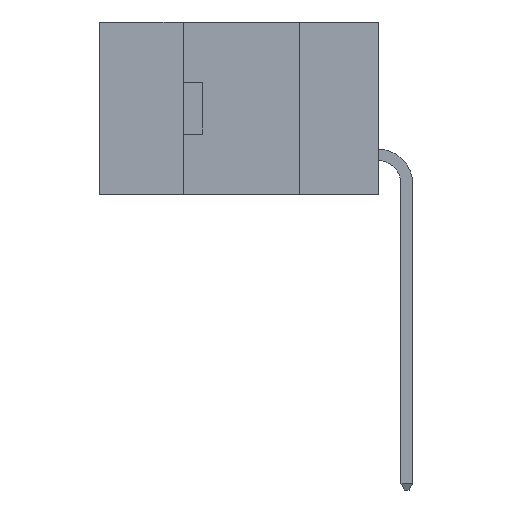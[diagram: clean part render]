
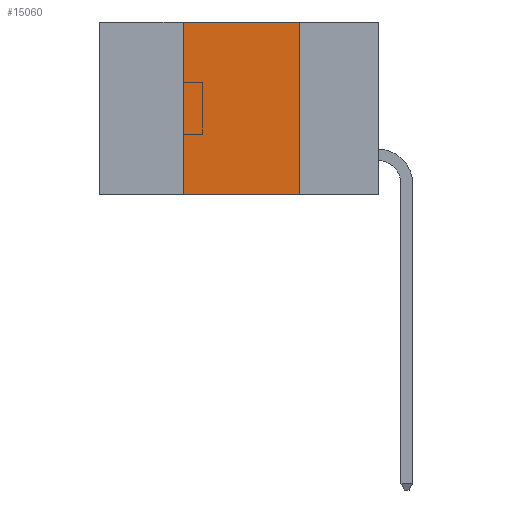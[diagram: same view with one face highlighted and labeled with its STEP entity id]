
A CAD part, left-side view. The second image highlights one B-rep face of the part: STEP entity #15060.
In plain terms, the highlighted planar face has unit normal (-1, 0, 0).
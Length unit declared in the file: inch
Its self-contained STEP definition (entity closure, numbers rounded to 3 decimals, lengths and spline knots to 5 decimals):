
#1055 = CARTESIAN_POINT ( 'NONE',  ( 0., 0.17, 0. ) ) ;
#1073 = DIRECTION ( 'NONE',  ( 0., 0., 1. ) ) ;
#2686 = LINE ( 'NONE', #26273, #6857 ) ;
#3085 = LINE ( 'NONE', #21431, #13430 ) ;
#3296 = FACE_OUTER_BOUND ( 'NONE', #6291, .T. ) ;
#3690 = ORIENTED_EDGE ( 'NONE', *, *, #23099, .T. ) ;
#4072 = VECTOR ( 'NONE', #1073, 39.37008 ) ;
#4460 = EDGE_CURVE ( 'NONE', #14767, #19851, #20591, .T. ) ;
#4537 = DIRECTION ( 'NONE',  ( 0., 0., -1. ) ) ;
#5478 = DIRECTION ( 'NONE',  ( 0., -1., 0. ) ) ;
#6291 = EDGE_LOOP ( 'NONE', ( #19590, #8863, #16906, #3690 ) ) ;
#6857 = VECTOR ( 'NONE', #16067, 39.37008 ) ;
#8240 = EDGE_CURVE ( 'NONE', #21150, #10638, #3085, .T. ) ;
#8863 = ORIENTED_EDGE ( 'NONE', *, *, #14691, .F. ) ;
#8996 = DIRECTION ( 'NONE',  ( 0., 0., -1. ) ) ;
#9226 = CARTESIAN_POINT ( 'NONE',  ( 0., 0.42, -0.37 ) ) ;
#10638 = VERTEX_POINT ( 'NONE', #18844 ) ;
#11165 = CARTESIAN_POINT ( 'NONE',  ( 0., 0.42, 0. ) ) ;
#12381 = AXIS2_PLACEMENT_3D ( 'NONE', #12777, #16963, #4537 ) ;
#12777 = CARTESIAN_POINT ( 'NONE',  ( 0., 0.6, 0. ) ) ;
#13008 = LINE ( 'NONE', #15803, #23344 ) ;
#13430 = VECTOR ( 'NONE', #8996, 39.37008 ) ;
#14691 = EDGE_CURVE ( 'NONE', #19851, #21150, #13008, .T. ) ;
#14767 = VERTEX_POINT ( 'NONE', #24260 ) ;
#14860 = PLANE ( 'NONE',  #12381 ) ;
#15060 = ADVANCED_FACE ( 'NONE', ( #3296 ), #14860, .F. ) ;
#15803 = CARTESIAN_POINT ( 'NONE',  ( 0., 0.6, 0. ) ) ;
#16067 = DIRECTION ( 'NONE',  ( 0., -1., 0. ) ) ;
#16906 = ORIENTED_EDGE ( 'NONE', *, *, #4460, .F. ) ;
#16963 = DIRECTION ( 'NONE',  ( 1., 0., 0. ) ) ;
#18844 = CARTESIAN_POINT ( 'NONE',  ( 0., 0.17, -0.37 ) ) ;
#19590 = ORIENTED_EDGE ( 'NONE', *, *, #8240, .F. ) ;
#19851 = VERTEX_POINT ( 'NONE', #11165 ) ;
#20591 = LINE ( 'NONE', #9226, #4072 ) ;
#21150 = VERTEX_POINT ( 'NONE', #1055 ) ;
#21431 = CARTESIAN_POINT ( 'NONE',  ( 0., 0.17, -0.37 ) ) ;
#23099 = EDGE_CURVE ( 'NONE', #14767, #10638, #2686, .T. ) ;
#23344 = VECTOR ( 'NONE', #5478, 39.37008 ) ;
#24260 = CARTESIAN_POINT ( 'NONE',  ( 0., 0.42, -0.37 ) ) ;
#26273 = CARTESIAN_POINT ( 'NONE',  ( 0., 0.6, -0.37 ) ) ;
